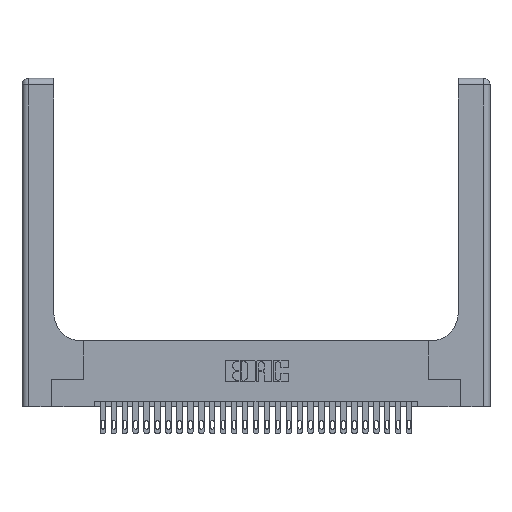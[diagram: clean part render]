
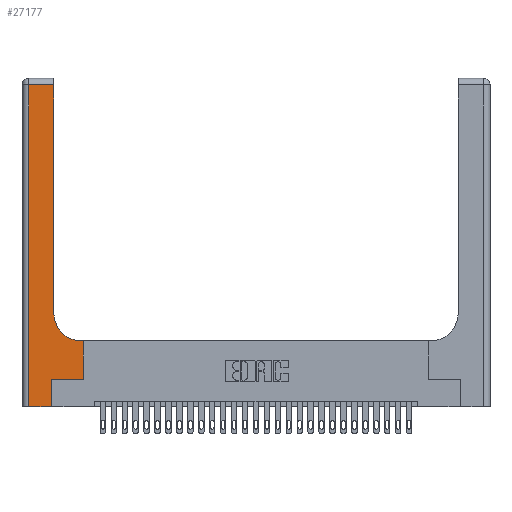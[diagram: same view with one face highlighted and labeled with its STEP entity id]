
A CAD part, top view. The second image highlights one B-rep face of the part: STEP entity #27177.
In plain terms, the highlighted planar face has unit normal (0, 0, 1).
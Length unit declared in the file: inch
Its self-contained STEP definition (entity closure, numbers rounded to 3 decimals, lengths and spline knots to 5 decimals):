
#303 = EDGE_LOOP ( 'NONE', ( #25473, #7362, #26281, #25428, #8467, #10229, #6136, #2146, #5436 ) ) ;
#627 = CARTESIAN_POINT ( 'NONE',  ( 0.2915, 2.94, 0.37 ) ) ;
#703 = EDGE_CURVE ( 'NONE', #17091, #9751, #28935, .T. ) ;
#1311 = AXIS2_PLACEMENT_3D ( 'NONE', #16049, #25259, #22914 ) ;
#1723 = VERTEX_POINT ( 'NONE', #627 ) ;
#1806 = EDGE_CURVE ( 'NONE', #1723, #13317, #24479, .T. ) ;
#2146 = ORIENTED_EDGE ( 'NONE', *, *, #19598, .T. ) ;
#2840 = DIRECTION ( 'NONE',  ( 0., -1., 0. ) ) ;
#3111 = EDGE_CURVE ( 'NONE', #14888, #18772, #19492, .T. ) ;
#3449 = VERTEX_POINT ( 'NONE', #5306 ) ;
#3759 = DIRECTION ( 'NONE',  ( -1., 0., 0. ) ) ;
#4265 = VECTOR ( 'NONE', #19721, 39.37008 ) ;
#4929 = CARTESIAN_POINT ( 'NONE',  ( 0.06, 0., 0.37 ) ) ;
#5306 = CARTESIAN_POINT ( 'NONE',  ( 0.269, 0., 0.37 ) ) ;
#5436 = ORIENTED_EDGE ( 'NONE', *, *, #3111, .T. ) ;
#5602 = CARTESIAN_POINT ( 'NONE',  ( 0.06, 2.94, 0.37 ) ) ;
#5917 = CARTESIAN_POINT ( 'NONE',  ( 0.269, 0., 0.37 ) ) ;
#6136 = ORIENTED_EDGE ( 'NONE', *, *, #703, .T. ) ;
#6375 = AXIS2_PLACEMENT_3D ( 'NONE', #11820, #9733, #11926 ) ;
#6436 = VECTOR ( 'NONE', #9882, 39.37008 ) ;
#7286 = EDGE_CURVE ( 'NONE', #23542, #3449, #14967, .T. ) ;
#7362 = ORIENTED_EDGE ( 'NONE', *, *, #1806, .T. ) ;
#8242 = DIRECTION ( 'NONE',  ( 0., 1., 0. ) ) ;
#8467 = ORIENTED_EDGE ( 'NONE', *, *, #15550, .T. ) ;
#9485 = CARTESIAN_POINT ( 'NONE',  ( 0., 0., 0.37 ) ) ;
#9528 = PLANE ( 'NONE',  #6375 ) ;
#9733 = DIRECTION ( 'NONE',  ( 0., 0., -1. ) ) ;
#9751 = VERTEX_POINT ( 'NONE', #18973 ) ;
#9882 = DIRECTION ( 'NONE',  ( -1., 0., 0. ) ) ;
#10124 = VECTOR ( 'NONE', #17617, 39.37008 ) ;
#10229 = ORIENTED_EDGE ( 'NONE', *, *, #24446, .T. ) ;
#10924 = VECTOR ( 'NONE', #8242, 39.37008 ) ;
#11820 = CARTESIAN_POINT ( 'NONE',  ( 0., 3., 0.37 ) ) ;
#11909 = VECTOR ( 'NONE', #2840, 39.37008 ) ;
#11926 = DIRECTION ( 'NONE',  ( -1., 0., 0. ) ) ;
#13317 = VERTEX_POINT ( 'NONE', #5602 ) ;
#13887 = DIRECTION ( 'NONE',  ( 1., 0., 0. ) ) ;
#14121 = CARTESIAN_POINT ( 'NONE',  ( 0.2915, 3., 0.37 ) ) ;
#14449 = LINE ( 'NONE', #14121, #18740 ) ;
#14797 = LINE ( 'NONE', #18804, #11909 ) ;
#14888 = VERTEX_POINT ( 'NONE', #24317 ) ;
#14967 = LINE ( 'NONE', #9485, #25607 ) ;
#15550 = EDGE_CURVE ( 'NONE', #3449, #25186, #18785, .T. ) ;
#16049 = CARTESIAN_POINT ( 'NONE',  ( 0.5415, 0.85, 0.37 ) ) ;
#16735 = EDGE_CURVE ( 'NONE', #18772, #1723, #14449, .T. ) ;
#16996 = CARTESIAN_POINT ( 'NONE',  ( 0.2915, 0.6, 0.37 ) ) ;
#17091 = VERTEX_POINT ( 'NONE', #24224 ) ;
#17115 = CARTESIAN_POINT ( 'NONE',  ( 0.2915, 0.85, 0.37 ) ) ;
#17617 = DIRECTION ( 'NONE',  ( 1., 0., 0. ) ) ;
#18740 = VECTOR ( 'NONE', #27621, 39.37008 ) ;
#18772 = VERTEX_POINT ( 'NONE', #17115 ) ;
#18785 = LINE ( 'NONE', #5917, #10924 ) ;
#18804 = CARTESIAN_POINT ( 'NONE',  ( 0.06, 3., 0.37 ) ) ;
#18973 = CARTESIAN_POINT ( 'NONE',  ( 0.5585, 0.6, 0.37 ) ) ;
#19411 = LINE ( 'NONE', #22293, #10124 ) ;
#19492 = CIRCLE ( 'NONE', #1311, 0.25 ) ;
#19598 = EDGE_CURVE ( 'NONE', #9751, #14888, #25019, .T. ) ;
#19721 = DIRECTION ( 'NONE',  ( 0., 1., 0. ) ) ;
#19903 = VECTOR ( 'NONE', #3759, 39.37008 ) ;
#22293 = CARTESIAN_POINT ( 'NONE',  ( 0.269, 0.25, 0.37 ) ) ;
#22847 = CARTESIAN_POINT ( 'NONE',  ( 0.269, 0.25, 0.37 ) ) ;
#22914 = DIRECTION ( 'NONE',  ( 1., 0., 0. ) ) ;
#23542 = VERTEX_POINT ( 'NONE', #4929 ) ;
#24195 = EDGE_CURVE ( 'NONE', #13317, #23542, #14797, .T. ) ;
#24224 = CARTESIAN_POINT ( 'NONE',  ( 0.5585, 0.25, 0.37 ) ) ;
#24317 = CARTESIAN_POINT ( 'NONE',  ( 0.5415, 0.6, 0.37 ) ) ;
#24347 = CARTESIAN_POINT ( 'NONE',  ( 0.5585, 0.25, 0.37 ) ) ;
#24446 = EDGE_CURVE ( 'NONE', #25186, #17091, #19411, .T. ) ;
#24479 = LINE ( 'NONE', #28744, #19903 ) ;
#24981 = FACE_OUTER_BOUND ( 'NONE', #303, .T. ) ;
#25019 = LINE ( 'NONE', #16996, #6436 ) ;
#25186 = VERTEX_POINT ( 'NONE', #22847 ) ;
#25259 = DIRECTION ( 'NONE',  ( 0., 0., -1. ) ) ;
#25428 = ORIENTED_EDGE ( 'NONE', *, *, #7286, .T. ) ;
#25473 = ORIENTED_EDGE ( 'NONE', *, *, #16735, .T. ) ;
#25607 = VECTOR ( 'NONE', #13887, 39.37008 ) ;
#26281 = ORIENTED_EDGE ( 'NONE', *, *, #24195, .T. ) ;
#27177 = ADVANCED_FACE ( 'NONE', ( #24981 ), #9528, .F. ) ;
#27621 = DIRECTION ( 'NONE',  ( 0., 1., 0. ) ) ;
#28744 = CARTESIAN_POINT ( 'NONE',  ( 0., 2.94, 0.37 ) ) ;
#28935 = LINE ( 'NONE', #24347, #4265 ) ;
